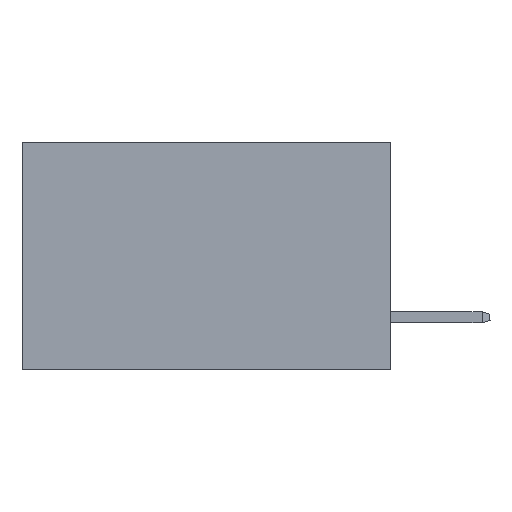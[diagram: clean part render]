
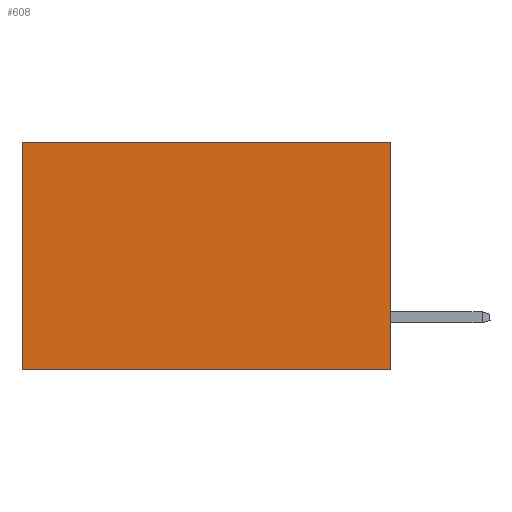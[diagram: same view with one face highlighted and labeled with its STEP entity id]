
A CAD part, left-side view. The second image highlights one B-rep face of the part: STEP entity #608.
In plain terms, the highlighted planar face has unit normal (-1, 0, 0).
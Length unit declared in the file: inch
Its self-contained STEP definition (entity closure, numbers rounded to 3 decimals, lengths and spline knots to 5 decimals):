
#608 = ADVANCED_FACE ( 'NONE', ( #11182 ), #33896, .F. ) ;
#686 = VECTOR ( 'NONE', #25007, 39.37008 ) ;
#3299 = DIRECTION ( 'NONE',  ( 0., 1., 0. ) ) ;
#3496 = DIRECTION ( 'NONE',  ( 1., 0., 0. ) ) ;
#5935 = VERTEX_POINT ( 'NONE', #27907 ) ;
#6258 = VERTEX_POINT ( 'NONE', #14105 ) ;
#6769 = CARTESIAN_POINT ( 'NONE',  ( 0.2875, 0., 0. ) ) ;
#7069 = EDGE_LOOP ( 'NONE', ( #36898, #35989, #17241, #14355 ) ) ;
#7956 = LINE ( 'NONE', #6769, #686 ) ;
#10413 = CARTESIAN_POINT ( 'NONE',  ( 0.2875, 0., 0. ) ) ;
#10467 = LINE ( 'NONE', #10413, #24681 ) ;
#11182 = FACE_OUTER_BOUND ( 'NONE', #7069, .T. ) ;
#12157 = VERTEX_POINT ( 'NONE', #31219 ) ;
#13483 = CARTESIAN_POINT ( 'NONE',  ( 0.2875, 0.6, 0. ) ) ;
#13490 = DIRECTION ( 'NONE',  ( 0., 0., -1. ) ) ;
#14105 = CARTESIAN_POINT ( 'NONE',  ( 0.2875, 0.6, 0. ) ) ;
#14355 = ORIENTED_EDGE ( 'NONE', *, *, #27460, .T. ) ;
#17241 = ORIENTED_EDGE ( 'NONE', *, *, #34412, .F. ) ;
#17313 = AXIS2_PLACEMENT_3D ( 'NONE', #25778, #3496, #20147 ) ;
#20147 = DIRECTION ( 'NONE',  ( 0., 0., -1. ) ) ;
#20533 = DIRECTION ( 'NONE',  ( 0., 0., -1. ) ) ;
#21582 = CARTESIAN_POINT ( 'NONE',  ( 0.2875, 0., -0.37 ) ) ;
#22941 = LINE ( 'NONE', #21582, #23903 ) ;
#23059 = VECTOR ( 'NONE', #20533, 39.37008 ) ;
#23903 = VECTOR ( 'NONE', #3299, 39.37008 ) ;
#24308 = VERTEX_POINT ( 'NONE', #36108 ) ;
#24681 = VECTOR ( 'NONE', #13490, 39.37008 ) ;
#25007 = DIRECTION ( 'NONE',  ( 0., 1., 0. ) ) ;
#25778 = CARTESIAN_POINT ( 'NONE',  ( 0.2875, 0., 0. ) ) ;
#27460 = EDGE_CURVE ( 'NONE', #24308, #6258, #7956, .T. ) ;
#27907 = CARTESIAN_POINT ( 'NONE',  ( 0.2875, 0.6, -0.37 ) ) ;
#30099 = EDGE_CURVE ( 'NONE', #12157, #5935, #22941, .T. ) ;
#31219 = CARTESIAN_POINT ( 'NONE',  ( 0.2875, 0., -0.37 ) ) ;
#32122 = LINE ( 'NONE', #13483, #23059 ) ;
#33896 = PLANE ( 'NONE',  #17313 ) ;
#34412 = EDGE_CURVE ( 'NONE', #24308, #12157, #10467, .T. ) ;
#35989 = ORIENTED_EDGE ( 'NONE', *, *, #30099, .F. ) ;
#36108 = CARTESIAN_POINT ( 'NONE',  ( 0.2875, 0., 0. ) ) ;
#36368 = EDGE_CURVE ( 'NONE', #6258, #5935, #32122, .T. ) ;
#36898 = ORIENTED_EDGE ( 'NONE', *, *, #36368, .T. ) ;
